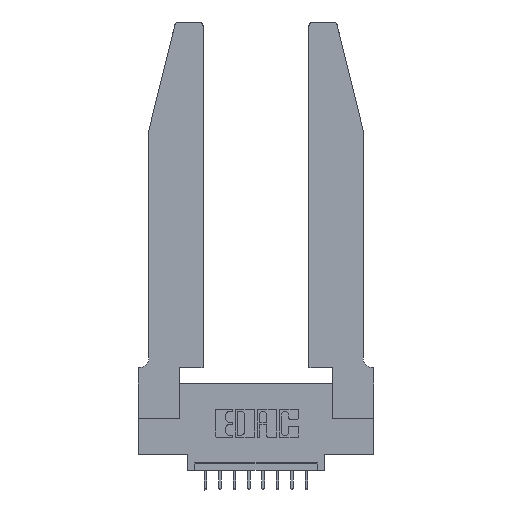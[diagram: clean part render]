
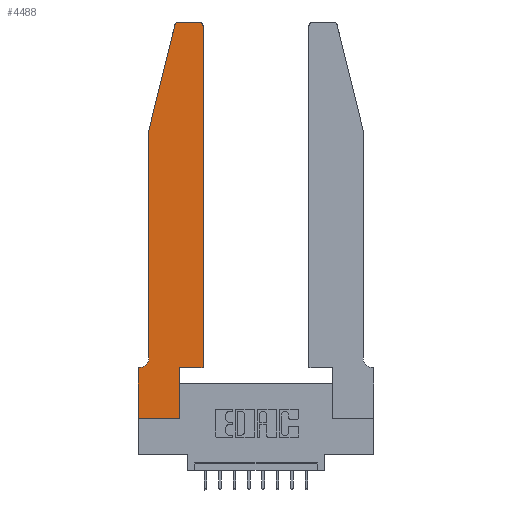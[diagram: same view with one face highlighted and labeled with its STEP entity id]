
A CAD part, top view. The second image highlights one B-rep face of the part: STEP entity #4488.
In plain terms, the highlighted planar face has unit normal (0, 0, 1).
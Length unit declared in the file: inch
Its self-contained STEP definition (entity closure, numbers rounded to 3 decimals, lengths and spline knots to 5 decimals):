
#196 = VECTOR ( 'NONE', #3082, 39.37008 ) ;
#301 = DIRECTION ( 'NONE',  ( 1., 0., 0. ) ) ;
#315 = CARTESIAN_POINT ( 'NONE',  ( 0., 0.35, 0.37 ) ) ;
#532 = EDGE_CURVE ( 'NONE', #1739, #4956, #6331, .T. ) ;
#599 = VERTEX_POINT ( 'NONE', #13131 ) ;
#676 = VECTOR ( 'NONE', #4485, 39.37008 ) ;
#733 = CARTESIAN_POINT ( 'NONE',  ( 0.0755, 0.35, 0.37 ) ) ;
#735 = VERTEX_POINT ( 'NONE', #9053 ) ;
#767 = CARTESIAN_POINT ( 'NONE',  ( 0.2865, 0., 0.37 ) ) ;
#814 = EDGE_CURVE ( 'NONE', #2778, #2300, #4358, .T. ) ;
#1035 = FACE_OUTER_BOUND ( 'NONE', #7782, .T. ) ;
#1302 = EDGE_CURVE ( 'NONE', #7468, #11114, #1569, .T. ) ;
#1436 = DIRECTION ( 'NONE',  ( 1., 0., 0. ) ) ;
#1544 = AXIS2_PLACEMENT_3D ( 'NONE', #10175, #7835, #12313 ) ;
#1569 = CIRCLE ( 'NONE', #3081, 0.03 ) ;
#1739 = VERTEX_POINT ( 'NONE', #4040 ) ;
#1832 = CARTESIAN_POINT ( 'NONE',  ( 0.284, 2.75, 0.37 ) ) ;
#1915 = LINE ( 'NONE', #733, #9925 ) ;
#2044 = CARTESIAN_POINT ( 'NONE',  ( 0.4505, 2.72, 0.37 ) ) ;
#2178 = CARTESIAN_POINT ( 'NONE',  ( 0.25487, 2.72718, 0.37 ) ) ;
#2300 = VERTEX_POINT ( 'NONE', #7114 ) ;
#2637 = DIRECTION ( 'NONE',  ( 0., 0., 1. ) ) ;
#2739 = VERTEX_POINT ( 'NONE', #1832 ) ;
#2778 = VERTEX_POINT ( 'NONE', #3391 ) ;
#2786 = DIRECTION ( 'NONE',  ( 0., 1., 0. ) ) ;
#2840 = DIRECTION ( 'NONE',  ( 0., 1., 0. ) ) ;
#3081 = AXIS2_PLACEMENT_3D ( 'NONE', #14656, #2637, #7191 ) ;
#3082 = DIRECTION ( 'NONE',  ( 1., 0., 0. ) ) ;
#3174 = CIRCLE ( 'NONE', #11944, 0.03 ) ;
#3213 = VECTOR ( 'NONE', #2840, 39.37008 ) ;
#3391 = CARTESIAN_POINT ( 'NONE',  ( 0., 0.35, 0.37 ) ) ;
#3775 = VERTEX_POINT ( 'NONE', #14417 ) ;
#3946 = CARTESIAN_POINT ( 'NONE',  ( 0.284, 2.72, 0.37 ) ) ;
#3993 = CARTESIAN_POINT ( 'NONE',  ( 0.4205, 2.75, 0.37 ) ) ;
#4040 = CARTESIAN_POINT ( 'NONE',  ( 0.0755, 0.42, 0.37 ) ) ;
#4146 = ORIENTED_EDGE ( 'NONE', *, *, #7153, .T. ) ;
#4312 = ORIENTED_EDGE ( 'NONE', *, *, #6137, .T. ) ;
#4358 = LINE ( 'NONE', #4439, #5332 ) ;
#4439 = CARTESIAN_POINT ( 'NONE',  ( 0., 0., 0.37 ) ) ;
#4485 = DIRECTION ( 'NONE',  ( -0.239, -0.971, 0. ) ) ;
#4488 = ADVANCED_FACE ( 'NONE', ( #1035 ), #10686, .T. ) ;
#4525 = ORIENTED_EDGE ( 'NONE', *, *, #532, .T. ) ;
#4634 = ORIENTED_EDGE ( 'NONE', *, *, #10356, .T. ) ;
#4956 = VERTEX_POINT ( 'NONE', #15228 ) ;
#4990 = DIRECTION ( 'NONE',  ( 0., 0., 1. ) ) ;
#4994 = CARTESIAN_POINT ( 'NONE',  ( 0.4505, 0.35, 0.37 ) ) ;
#5332 = VECTOR ( 'NONE', #5466, 39.37008 ) ;
#5370 = ORIENTED_EDGE ( 'NONE', *, *, #6189, .T. ) ;
#5466 = DIRECTION ( 'NONE',  ( 0., -1., 0. ) ) ;
#6020 = CARTESIAN_POINT ( 'NONE',  ( 0.4505, 0.35, 0.37 ) ) ;
#6137 = EDGE_CURVE ( 'NONE', #7844, #599, #13584, .T. ) ;
#6189 = EDGE_CURVE ( 'NONE', #2739, #11957, #3174, .T. ) ;
#6331 = CIRCLE ( 'NONE', #1544, 0.07 ) ;
#6449 = CARTESIAN_POINT ( 'NONE',  ( 0.0755, 2., 0.37 ) ) ;
#6554 = LINE ( 'NONE', #11622, #196 ) ;
#6782 = VECTOR ( 'NONE', #9567, 39.37008 ) ;
#6876 = DIRECTION ( 'NONE',  ( -1., 0., 0. ) ) ;
#6948 = LINE ( 'NONE', #6020, #13657 ) ;
#7114 = CARTESIAN_POINT ( 'NONE',  ( 0., 0., 0.37 ) ) ;
#7153 = EDGE_CURVE ( 'NONE', #599, #3775, #6948, .T. ) ;
#7191 = DIRECTION ( 'NONE',  ( 1., 0., 0. ) ) ;
#7286 = EDGE_CURVE ( 'NONE', #3775, #7468, #12273, .T. ) ;
#7468 = VERTEX_POINT ( 'NONE', #2044 ) ;
#7590 = CARTESIAN_POINT ( 'NONE',  ( 0.0755, 2., 0.37 ) ) ;
#7598 = ORIENTED_EDGE ( 'NONE', *, *, #814, .T. ) ;
#7612 = LINE ( 'NONE', #6449, #676 ) ;
#7782 = EDGE_LOOP ( 'NONE', ( #8257, #5370, #4634, #13661, #4525, #10797, #7598, #8283, #4312, #4146, #12829, #9149 ) ) ;
#7835 = DIRECTION ( 'NONE',  ( 0., 0., -1. ) ) ;
#7844 = VERTEX_POINT ( 'NONE', #767 ) ;
#8045 = EDGE_CURVE ( 'NONE', #735, #1739, #8853, .T. ) ;
#8178 = EDGE_CURVE ( 'NONE', #4956, #2778, #1915, .T. ) ;
#8257 = ORIENTED_EDGE ( 'NONE', *, *, #15289, .T. ) ;
#8283 = ORIENTED_EDGE ( 'NONE', *, *, #13147, .T. ) ;
#8317 = CARTESIAN_POINT ( 'NONE',  ( 0.2605, 2.75, 0.37 ) ) ;
#8402 = VECTOR ( 'NONE', #14983, 39.37008 ) ;
#8853 = LINE ( 'NONE', #7590, #8402 ) ;
#9053 = CARTESIAN_POINT ( 'NONE',  ( 0.0755, 2., 0.37 ) ) ;
#9149 = ORIENTED_EDGE ( 'NONE', *, *, #1302, .T. ) ;
#9415 = LINE ( 'NONE', #8317, #6782 ) ;
#9567 = DIRECTION ( 'NONE',  ( -1., 0., 0. ) ) ;
#9925 = VECTOR ( 'NONE', #6876, 39.37008 ) ;
#10048 = DIRECTION ( 'NONE',  ( 0., 0., 1. ) ) ;
#10147 = AXIS2_PLACEMENT_3D ( 'NONE', #315, #4990, #1436 ) ;
#10175 = CARTESIAN_POINT ( 'NONE',  ( 0.0055, 0.42, 0.37 ) ) ;
#10356 = EDGE_CURVE ( 'NONE', #11957, #735, #7612, .T. ) ;
#10686 = PLANE ( 'NONE',  #10147 ) ;
#10797 = ORIENTED_EDGE ( 'NONE', *, *, #8178, .T. ) ;
#11114 = VERTEX_POINT ( 'NONE', #3993 ) ;
#11622 = CARTESIAN_POINT ( 'NONE',  ( 0., 0., 0.37 ) ) ;
#11944 = AXIS2_PLACEMENT_3D ( 'NONE', #3946, #10048, #301 ) ;
#11957 = VERTEX_POINT ( 'NONE', #2178 ) ;
#12273 = LINE ( 'NONE', #4994, #12921 ) ;
#12313 = DIRECTION ( 'NONE',  ( -1., 0., 0. ) ) ;
#12829 = ORIENTED_EDGE ( 'NONE', *, *, #7286, .T. ) ;
#12921 = VECTOR ( 'NONE', #2786, 39.37008 ) ;
#12982 = DIRECTION ( 'NONE',  ( 1., 0., 0. ) ) ;
#13131 = CARTESIAN_POINT ( 'NONE',  ( 0.2865, 0.35, 0.37 ) ) ;
#13147 = EDGE_CURVE ( 'NONE', #2300, #7844, #6554, .T. ) ;
#13584 = LINE ( 'NONE', #14706, #3213 ) ;
#13657 = VECTOR ( 'NONE', #12982, 39.37008 ) ;
#13661 = ORIENTED_EDGE ( 'NONE', *, *, #8045, .T. ) ;
#14417 = CARTESIAN_POINT ( 'NONE',  ( 0.4505, 0.35, 0.37 ) ) ;
#14656 = CARTESIAN_POINT ( 'NONE',  ( 0.4205, 2.72, 0.37 ) ) ;
#14706 = CARTESIAN_POINT ( 'NONE',  ( 0.2865, 0.35, 0.37 ) ) ;
#14983 = DIRECTION ( 'NONE',  ( 0., -1., 0. ) ) ;
#15228 = CARTESIAN_POINT ( 'NONE',  ( 0.0055, 0.35, 0.37 ) ) ;
#15289 = EDGE_CURVE ( 'NONE', #11114, #2739, #9415, .T. ) ;
